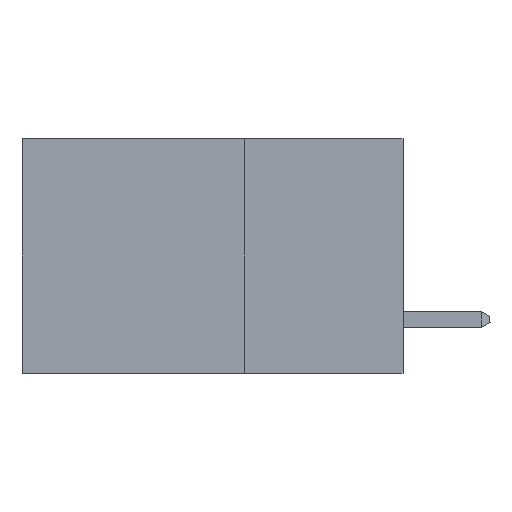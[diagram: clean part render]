
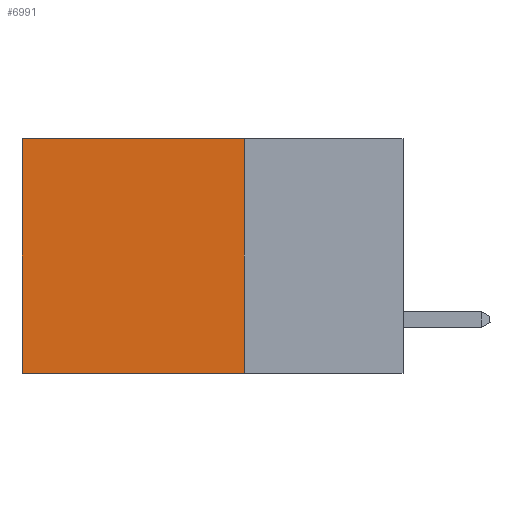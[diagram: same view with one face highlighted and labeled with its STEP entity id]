
A CAD part, left-side view. The second image highlights one B-rep face of the part: STEP entity #6991.
In plain terms, the highlighted planar face has unit normal (-1, 0, 0).
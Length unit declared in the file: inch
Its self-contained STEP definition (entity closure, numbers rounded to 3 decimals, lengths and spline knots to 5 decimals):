
#835 = CARTESIAN_POINT ( 'NONE',  ( 0.2875, 0.25, 0. ) ) ;
#1762 = LINE ( 'NONE', #7088, #5177 ) ;
#2837 = CARTESIAN_POINT ( 'NONE',  ( 0.2875, 0.6, 0. ) ) ;
#3113 = VERTEX_POINT ( 'NONE', #21133 ) ;
#4659 = LINE ( 'NONE', #7931, #7705 ) ;
#4937 = EDGE_CURVE ( 'NONE', #3113, #34426, #9954, .T. ) ;
#5177 = VECTOR ( 'NONE', #15134, 39.37008 ) ;
#5626 = DIRECTION ( 'NONE',  ( 1., 0., 0. ) ) ;
#5720 = DIRECTION ( 'NONE',  ( 0., 0., -1. ) ) ;
#6991 = ADVANCED_FACE ( 'NONE', ( #22964 ), #16860, .F. ) ;
#7088 = CARTESIAN_POINT ( 'NONE',  ( 0.2875, 0.6, 0. ) ) ;
#7705 = VECTOR ( 'NONE', #26992, 39.37008 ) ;
#7931 = CARTESIAN_POINT ( 'NONE',  ( 0.2875, 0.25, -0.37 ) ) ;
#9954 = LINE ( 'NONE', #835, #33335 ) ;
#12909 = VERTEX_POINT ( 'NONE', #20859 ) ;
#15134 = DIRECTION ( 'NONE',  ( 0., 0., -1. ) ) ;
#15824 = AXIS2_PLACEMENT_3D ( 'NONE', #22222, #5626, #5720 ) ;
#16860 = PLANE ( 'NONE',  #15824 ) ;
#17194 = EDGE_CURVE ( 'NONE', #29691, #12909, #1762, .T. ) ;
#17413 = CARTESIAN_POINT ( 'NONE',  ( 0.2875, 0.25, 0. ) ) ;
#17653 = ORIENTED_EDGE ( 'NONE', *, *, #26404, .T. ) ;
#19827 = EDGE_CURVE ( 'NONE', #34426, #12909, #4659, .T. ) ;
#20834 = VECTOR ( 'NONE', #28611, 39.37008 ) ;
#20859 = CARTESIAN_POINT ( 'NONE',  ( 0.2875, 0.6, -0.37 ) ) ;
#21133 = CARTESIAN_POINT ( 'NONE',  ( 0.2875, 0.25, 0. ) ) ;
#22222 = CARTESIAN_POINT ( 'NONE',  ( 0.2875, 0.25, 0. ) ) ;
#22964 = FACE_OUTER_BOUND ( 'NONE', #28727, .T. ) ;
#23009 = CARTESIAN_POINT ( 'NONE',  ( 0.2875, 0.25, -0.37 ) ) ;
#25804 = DIRECTION ( 'NONE',  ( 0., 0., -1. ) ) ;
#26169 = ORIENTED_EDGE ( 'NONE', *, *, #17194, .T. ) ;
#26404 = EDGE_CURVE ( 'NONE', #3113, #29691, #28050, .T. ) ;
#26992 = DIRECTION ( 'NONE',  ( 0., 1., 0. ) ) ;
#28050 = LINE ( 'NONE', #17413, #20834 ) ;
#28611 = DIRECTION ( 'NONE',  ( 0., 1., 0. ) ) ;
#28727 = EDGE_LOOP ( 'NONE', ( #26169, #34395, #33680, #17653 ) ) ;
#29691 = VERTEX_POINT ( 'NONE', #2837 ) ;
#33335 = VECTOR ( 'NONE', #25804, 39.37008 ) ;
#33680 = ORIENTED_EDGE ( 'NONE', *, *, #4937, .F. ) ;
#34395 = ORIENTED_EDGE ( 'NONE', *, *, #19827, .F. ) ;
#34426 = VERTEX_POINT ( 'NONE', #23009 ) ;
